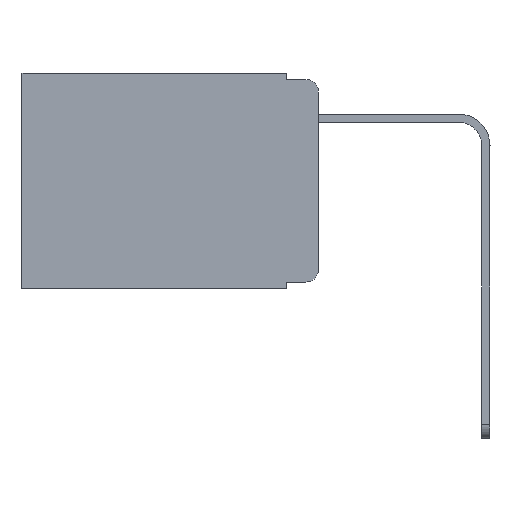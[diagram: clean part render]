
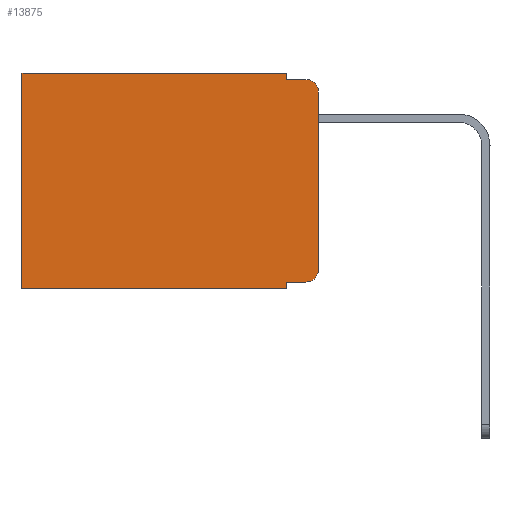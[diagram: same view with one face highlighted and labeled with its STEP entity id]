
A CAD part, left-side view. The second image highlights one B-rep face of the part: STEP entity #13875.
In plain terms, the highlighted planar face has unit normal (-1, 0, 0).
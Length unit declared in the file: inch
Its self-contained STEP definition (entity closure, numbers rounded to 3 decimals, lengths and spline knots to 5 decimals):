
#566 = ORIENTED_EDGE ( 'NONE', *, *, #16466, .T. ) ;
#756 = VERTEX_POINT ( 'NONE', #18680 ) ;
#897 = LINE ( 'NONE', #11280, #21768 ) ;
#1265 = DIRECTION ( 'NONE',  ( 0., 0., -1. ) ) ;
#1351 = DIRECTION ( 'NONE',  ( -1., 0., 0. ) ) ;
#1383 = VERTEX_POINT ( 'NONE', #15745 ) ;
#1418 = CARTESIAN_POINT ( 'NONE',  ( 0.298, 0., -0.343 ) ) ;
#2138 = CARTESIAN_POINT ( 'NONE',  ( 0.298, 0.473, -0.343 ) ) ;
#2436 = EDGE_CURVE ( 'NONE', #1383, #2443, #7845, .T. ) ;
#2443 = VERTEX_POINT ( 'NONE', #5019 ) ;
#2965 = VECTOR ( 'NONE', #17710, 39.37008 ) ;
#3221 = EDGE_CURVE ( 'NONE', #756, #11797, #17431, .T. ) ;
#3241 = ORIENTED_EDGE ( 'NONE', *, *, #2436, .F. ) ;
#3385 = VERTEX_POINT ( 'NONE', #13504 ) ;
#3472 = VERTEX_POINT ( 'NONE', #17965 ) ;
#4570 = PLANE ( 'NONE',  #21347 ) ;
#4859 = EDGE_CURVE ( 'NONE', #3472, #14589, #22074, .T. ) ;
#5019 = CARTESIAN_POINT ( 'NONE',  ( 0.298, 0., -0.313 ) ) ;
#5186 = VECTOR ( 'NONE', #21382, 39.37008 ) ;
#5737 = ORIENTED_EDGE ( 'NONE', *, *, #13944, .F. ) ;
#5836 = DIRECTION ( 'NONE',  ( 0., 0., -1. ) ) ;
#6185 = FACE_OUTER_BOUND ( 'NONE', #12712, .T. ) ;
#7199 = CARTESIAN_POINT ( 'NONE',  ( 0.298, 0.473, 0. ) ) ;
#7666 = CIRCLE ( 'NONE', #22510, 0.02 ) ;
#7845 = LINE ( 'NONE', #10795, #22456 ) ;
#7858 = DIRECTION ( 'NONE',  ( 0., 1., 0. ) ) ;
#8232 = DIRECTION ( 'NONE',  ( 1., 0., 0. ) ) ;
#8437 = CARTESIAN_POINT ( 'NONE',  ( 0.298, 0.02, -0.333 ) ) ;
#9373 = DIRECTION ( 'NONE',  ( 0., 0., -1. ) ) ;
#9549 = VERTEX_POINT ( 'NONE', #14775 ) ;
#10428 = DIRECTION ( 'NONE',  ( 0., 0., -1. ) ) ;
#10795 = CARTESIAN_POINT ( 'NONE',  ( 0.298, 0., 0. ) ) ;
#10944 = VERTEX_POINT ( 'NONE', #22520 ) ;
#11280 = CARTESIAN_POINT ( 'NONE',  ( 0.298, 0., 0. ) ) ;
#11348 = VECTOR ( 'NONE', #9373, 39.37008 ) ;
#11797 = VERTEX_POINT ( 'NONE', #2138 ) ;
#11882 = EDGE_CURVE ( 'NONE', #13829, #10944, #897, .T. ) ;
#12126 = CARTESIAN_POINT ( 'NONE',  ( 0.298, 0.051, 0. ) ) ;
#12470 = CIRCLE ( 'NONE', #13433, 0.02 ) ;
#12486 = EDGE_CURVE ( 'NONE', #1383, #3385, #7666, .T. ) ;
#12712 = EDGE_LOOP ( 'NONE', ( #3241, #16640, #15465, #5737, #19976, #15364, #12938, #14184, #12718, #566 ) ) ;
#12718 = ORIENTED_EDGE ( 'NONE', *, *, #4859, .T. ) ;
#12938 = ORIENTED_EDGE ( 'NONE', *, *, #3221, .F. ) ;
#13433 = AXIS2_PLACEMENT_3D ( 'NONE', #21371, #1351, #21449 ) ;
#13504 = CARTESIAN_POINT ( 'NONE',  ( 0.298, 0.02, -0.01 ) ) ;
#13551 = CARTESIAN_POINT ( 'NONE',  ( 0.298, 0.051, 0. ) ) ;
#13829 = VERTEX_POINT ( 'NONE', #13551 ) ;
#13875 = ADVANCED_FACE ( 'NONE', ( #6185 ), #4570, .F. ) ;
#13944 = EDGE_CURVE ( 'NONE', #13829, #9549, #15285, .T. ) ;
#14184 = ORIENTED_EDGE ( 'NONE', *, *, #14930, .F. ) ;
#14284 = LINE ( 'NONE', #7199, #5186 ) ;
#14324 = EDGE_CURVE ( 'NONE', #9549, #3385, #21688, .T. ) ;
#14589 = VERTEX_POINT ( 'NONE', #8437 ) ;
#14746 = LINE ( 'NONE', #20143, #11348 ) ;
#14775 = CARTESIAN_POINT ( 'NONE',  ( 0.298, 0.051, -0.01 ) ) ;
#14867 = CARTESIAN_POINT ( 'NONE',  ( 0.298, 0.051, -0.333 ) ) ;
#14930 = EDGE_CURVE ( 'NONE', #3472, #756, #14746, .T. ) ;
#15285 = LINE ( 'NONE', #12126, #21696 ) ;
#15364 = ORIENTED_EDGE ( 'NONE', *, *, #22983, .T. ) ;
#15465 = ORIENTED_EDGE ( 'NONE', *, *, #14324, .F. ) ;
#15745 = CARTESIAN_POINT ( 'NONE',  ( 0.298, 0., -0.03 ) ) ;
#16137 = VECTOR ( 'NONE', #22199, 39.37008 ) ;
#16466 = EDGE_CURVE ( 'NONE', #14589, #2443, #12470, .T. ) ;
#16617 = CARTESIAN_POINT ( 'NONE',  ( 0.298, 0.051, -0.01 ) ) ;
#16640 = ORIENTED_EDGE ( 'NONE', *, *, #12486, .T. ) ;
#17347 = VECTOR ( 'NONE', #18763, 39.37008 ) ;
#17431 = LINE ( 'NONE', #1418, #2965 ) ;
#17710 = DIRECTION ( 'NONE',  ( 0., 1., 0. ) ) ;
#17965 = CARTESIAN_POINT ( 'NONE',  ( 0.298, 0.051, -0.333 ) ) ;
#18680 = CARTESIAN_POINT ( 'NONE',  ( 0.298, 0.051, -0.343 ) ) ;
#18763 = DIRECTION ( 'NONE',  ( 0., -1., 0. ) ) ;
#19031 = CARTESIAN_POINT ( 'NONE',  ( 0.298, 0., 0. ) ) ;
#19976 = ORIENTED_EDGE ( 'NONE', *, *, #11882, .T. ) ;
#20143 = CARTESIAN_POINT ( 'NONE',  ( 0.298, 0.051, 0. ) ) ;
#20816 = DIRECTION ( 'NONE',  ( 0., 0., -1. ) ) ;
#21347 = AXIS2_PLACEMENT_3D ( 'NONE', #19031, #8232, #20816 ) ;
#21371 = CARTESIAN_POINT ( 'NONE',  ( 0.298, 0.02, -0.313 ) ) ;
#21382 = DIRECTION ( 'NONE',  ( 0., 0., -1. ) ) ;
#21449 = DIRECTION ( 'NONE',  ( 0., 0., -1. ) ) ;
#21688 = LINE ( 'NONE', #16617, #16137 ) ;
#21696 = VECTOR ( 'NONE', #1265, 39.37008 ) ;
#21768 = VECTOR ( 'NONE', #7858, 39.37008 ) ;
#21989 = DIRECTION ( 'NONE',  ( -1., 0., 0. ) ) ;
#22074 = LINE ( 'NONE', #14867, #17347 ) ;
#22147 = CARTESIAN_POINT ( 'NONE',  ( 0.298, 0.02, -0.03 ) ) ;
#22199 = DIRECTION ( 'NONE',  ( 0., -1., 0. ) ) ;
#22456 = VECTOR ( 'NONE', #10428, 39.37008 ) ;
#22510 = AXIS2_PLACEMENT_3D ( 'NONE', #22147, #21989, #5836 ) ;
#22520 = CARTESIAN_POINT ( 'NONE',  ( 0.298, 0.473, 0. ) ) ;
#22983 = EDGE_CURVE ( 'NONE', #10944, #11797, #14284, .T. ) ;
